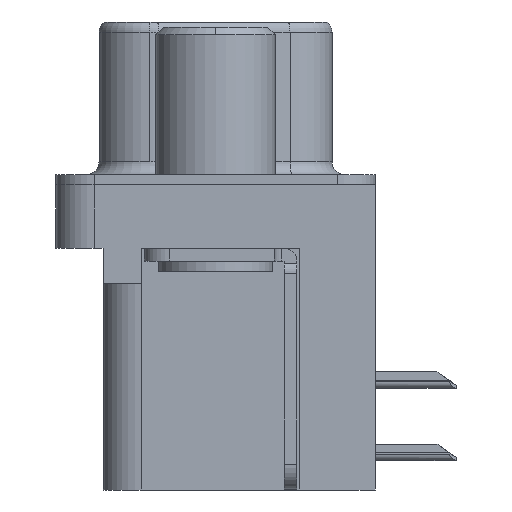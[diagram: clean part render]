
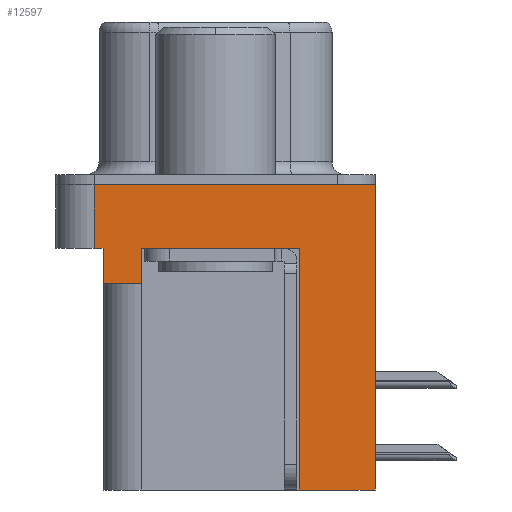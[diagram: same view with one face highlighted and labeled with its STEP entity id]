
A CAD part, left-side view. The second image highlights one B-rep face of the part: STEP entity #12597.
In plain terms, the highlighted planar face has unit normal (-1, 0, 0).
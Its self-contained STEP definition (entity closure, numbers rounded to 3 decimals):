
#607 = CARTESIAN_POINT ( 'NONE',  ( -2.91, 4.775, -2.5 ) ) ;
#899 = DIRECTION ( 'NONE',  ( 0., 1., 0. ) ) ;
#959 = CARTESIAN_POINT ( 'NONE',  ( -2.91, -3.295, -12. ) ) ;
#1027 = EDGE_CURVE ( 'NONE', #4445, #12948, #14519, .T. ) ;
#1030 = ORIENTED_EDGE ( 'NONE', *, *, #3721, .T. ) ;
#1157 = EDGE_CURVE ( 'NONE', #2964, #11732, #25582, .T. ) ;
#2090 = CARTESIAN_POINT ( 'NONE',  ( -2.91, -3.295, -2.5 ) ) ;
#2759 = ORIENTED_EDGE ( 'NONE', *, *, #10593, .F. ) ;
#2780 = CARTESIAN_POINT ( 'NONE',  ( -2.91, -6.275, -2.5 ) ) ;
#2907 = LINE ( 'NONE', #12152, #16195 ) ;
#2964 = VERTEX_POINT ( 'NONE', #18883 ) ;
#3447 = CARTESIAN_POINT ( 'NONE',  ( -2.91, 4.425, -3.9 ) ) ;
#3498 = LINE ( 'NONE', #16128, #26549 ) ;
#3721 = EDGE_CURVE ( 'NONE', #10003, #19166, #4699, .T. ) ;
#3926 = LINE ( 'NONE', #9504, #12039 ) ;
#3929 = VECTOR ( 'NONE', #26396, 1000. ) ;
#4445 = VERTEX_POINT ( 'NONE', #959 ) ;
#4699 = LINE ( 'NONE', #2780, #9532 ) ;
#4787 = VECTOR ( 'NONE', #15035, 1000. ) ;
#4850 = EDGE_CURVE ( 'NONE', #2964, #9743, #17274, .T. ) ;
#5217 = VERTEX_POINT ( 'NONE', #26245 ) ;
#5494 = PLANE ( 'NONE',  #21798 ) ;
#6623 = CARTESIAN_POINT ( 'NONE',  ( -2.91, 4.425, -2.5 ) ) ;
#7854 = DIRECTION ( 'NONE',  ( 0., -1., 0. ) ) ;
#8188 = DIRECTION ( 'NONE',  ( 0., 0., 1. ) ) ;
#8209 = ORIENTED_EDGE ( 'NONE', *, *, #1157, .T. ) ;
#8305 = CARTESIAN_POINT ( 'NONE',  ( -2.91, 2.895, -3.9 ) ) ;
#8582 = ORIENTED_EDGE ( 'NONE', *, *, #21553, .T. ) ;
#8649 = DIRECTION ( 'NONE',  ( 0., 0., 1. ) ) ;
#8750 = EDGE_CURVE ( 'NONE', #15251, #26075, #3926, .T. ) ;
#9006 = CARTESIAN_POINT ( 'NONE',  ( -2.91, -3.295, -12. ) ) ;
#9504 = CARTESIAN_POINT ( 'NONE',  ( -2.91, -6.275, -2.5 ) ) ;
#9532 = VECTOR ( 'NONE', #11100, 1000. ) ;
#9743 = VERTEX_POINT ( 'NONE', #23246 ) ;
#10003 = VERTEX_POINT ( 'NONE', #607 ) ;
#10593 = EDGE_CURVE ( 'NONE', #15251, #4445, #2907, .T. ) ;
#10845 = LINE ( 'NONE', #14287, #26807 ) ;
#11100 = DIRECTION ( 'NONE',  ( 0., -1., 0. ) ) ;
#11534 = ORIENTED_EDGE ( 'NONE', *, *, #25290, .F. ) ;
#11617 = DIRECTION ( 'NONE',  ( 0., 0., 1. ) ) ;
#11732 = VERTEX_POINT ( 'NONE', #26847 ) ;
#12039 = VECTOR ( 'NONE', #11617, 1000. ) ;
#12152 = CARTESIAN_POINT ( 'NONE',  ( -2.91, -3.295, -12. ) ) ;
#12597 = ADVANCED_FACE ( 'NONE', ( #16713 ), #5494, .T. ) ;
#12869 = ORIENTED_EDGE ( 'NONE', *, *, #13841, .F. ) ;
#12948 = VERTEX_POINT ( 'NONE', #2090 ) ;
#13212 = ORIENTED_EDGE ( 'NONE', *, *, #4850, .F. ) ;
#13841 = EDGE_CURVE ( 'NONE', #9743, #19166, #22433, .T. ) ;
#14287 = CARTESIAN_POINT ( 'NONE',  ( -2.91, 4.775, -2.5 ) ) ;
#14519 = LINE ( 'NONE', #9006, #4787 ) ;
#15035 = DIRECTION ( 'NONE',  ( 0., 0., 1. ) ) ;
#15251 = VERTEX_POINT ( 'NONE', #18044 ) ;
#15498 = VECTOR ( 'NONE', #8649, 1000. ) ;
#15724 = ORIENTED_EDGE ( 'NONE', *, *, #1027, .F. ) ;
#16014 = CARTESIAN_POINT ( 'NONE',  ( -2.91, -6.275, -2.5 ) ) ;
#16128 = CARTESIAN_POINT ( 'NONE',  ( -2.91, -6.275, 0. ) ) ;
#16195 = VECTOR ( 'NONE', #26426, 1000. ) ;
#16329 = EDGE_CURVE ( 'NONE', #5217, #26075, #3498, .T. ) ;
#16616 = EDGE_LOOP ( 'NONE', ( #18079, #11534, #1030, #12869, #13212, #8209, #8582, #15724, #2759, #18313 ) ) ;
#16713 = FACE_OUTER_BOUND ( 'NONE', #16616, .T. ) ;
#16837 = DIRECTION ( 'NONE',  ( 0., -1., 0. ) ) ;
#17274 = LINE ( 'NONE', #21770, #26756 ) ;
#18044 = CARTESIAN_POINT ( 'NONE',  ( -2.91, -6.275, -12. ) ) ;
#18079 = ORIENTED_EDGE ( 'NONE', *, *, #16329, .F. ) ;
#18313 = ORIENTED_EDGE ( 'NONE', *, *, #8750, .T. ) ;
#18599 = CARTESIAN_POINT ( 'NONE',  ( -2.91, -6.275, -2.5 ) ) ;
#18883 = CARTESIAN_POINT ( 'NONE',  ( -2.91, 2.895, -3.9 ) ) ;
#19166 = VERTEX_POINT ( 'NONE', #6623 ) ;
#19448 = LINE ( 'NONE', #18599, #21432 ) ;
#20212 = DIRECTION ( 'NONE',  ( 0., 0., 1. ) ) ;
#21432 = VECTOR ( 'NONE', #16837, 1000. ) ;
#21553 = EDGE_CURVE ( 'NONE', #11732, #12948, #19448, .T. ) ;
#21770 = CARTESIAN_POINT ( 'NONE',  ( -2.91, 4.425, -3.9 ) ) ;
#21798 = AXIS2_PLACEMENT_3D ( 'NONE', #16014, #24474, #20212 ) ;
#22433 = LINE ( 'NONE', #3447, #3929 ) ;
#23246 = CARTESIAN_POINT ( 'NONE',  ( -2.91, 4.425, -3.9 ) ) ;
#23621 = CARTESIAN_POINT ( 'NONE',  ( -2.91, -6.275, 0. ) ) ;
#24474 = DIRECTION ( 'NONE',  ( -1., 0., 0. ) ) ;
#25290 = EDGE_CURVE ( 'NONE', #10003, #5217, #10845, .T. ) ;
#25582 = LINE ( 'NONE', #8305, #15498 ) ;
#26075 = VERTEX_POINT ( 'NONE', #23621 ) ;
#26245 = CARTESIAN_POINT ( 'NONE',  ( -2.91, 4.775, 0. ) ) ;
#26396 = DIRECTION ( 'NONE',  ( 0., 0., 1. ) ) ;
#26426 = DIRECTION ( 'NONE',  ( 0., 1., 0. ) ) ;
#26549 = VECTOR ( 'NONE', #7854, 1000. ) ;
#26756 = VECTOR ( 'NONE', #899, 1000. ) ;
#26807 = VECTOR ( 'NONE', #8188, 1000. ) ;
#26847 = CARTESIAN_POINT ( 'NONE',  ( -2.91, 2.895, -2.5 ) ) ;
